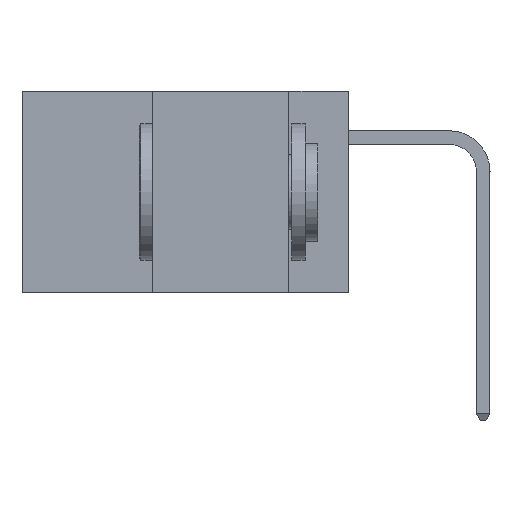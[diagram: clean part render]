
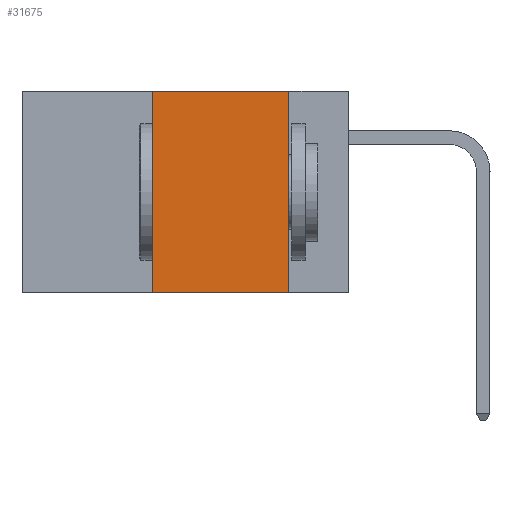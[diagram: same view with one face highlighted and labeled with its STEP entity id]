
A CAD part, left-side view. The second image highlights one B-rep face of the part: STEP entity #31675.
In plain terms, the highlighted planar face has unit normal (-1, 0, 0).
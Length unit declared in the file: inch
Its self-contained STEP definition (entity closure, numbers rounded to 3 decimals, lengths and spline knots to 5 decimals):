
#1002 = ORIENTED_EDGE ( 'NONE', *, *, #35847, .F. ) ;
#1972 = LINE ( 'NONE', #21958, #9373 ) ;
#2461 = LINE ( 'NONE', #11288, #18871 ) ;
#2498 = PLANE ( 'NONE',  #22065 ) ;
#6566 = CARTESIAN_POINT ( 'NONE',  ( 0., 0.36, -0.37 ) ) ;
#6732 = DIRECTION ( 'NONE',  ( 0., 0., -1. ) ) ;
#9373 = VECTOR ( 'NONE', #6732, 39.37008 ) ;
#9784 = VECTOR ( 'NONE', #36583, 39.37008 ) ;
#11142 = ORIENTED_EDGE ( 'NONE', *, *, #14828, .F. ) ;
#11288 = CARTESIAN_POINT ( 'NONE',  ( 0., 0.6, -0.37 ) ) ;
#11960 = DIRECTION ( 'NONE',  ( 0., 0., -1. ) ) ;
#13915 = CARTESIAN_POINT ( 'NONE',  ( 0., 0.36, 0. ) ) ;
#14675 = ORIENTED_EDGE ( 'NONE', *, *, #24342, .F. ) ;
#14828 = EDGE_CURVE ( 'NONE', #30409, #23588, #34005, .T. ) ;
#14893 = CARTESIAN_POINT ( 'NONE',  ( 0., 0.6, 0. ) ) ;
#16276 = DIRECTION ( 'NONE',  ( 0., 0., 1. ) ) ;
#17729 = VECTOR ( 'NONE', #16276, 39.37008 ) ;
#18871 = VECTOR ( 'NONE', #32500, 39.37008 ) ;
#19366 = CARTESIAN_POINT ( 'NONE',  ( 0., 0.11, -0.37 ) ) ;
#21958 = CARTESIAN_POINT ( 'NONE',  ( 0., 0.11, 0. ) ) ;
#22065 = AXIS2_PLACEMENT_3D ( 'NONE', #14893, #30103, #11960 ) ;
#23588 = VERTEX_POINT ( 'NONE', #36517 ) ;
#24342 = EDGE_CURVE ( 'NONE', #23588, #39618, #1972, .T. ) ;
#25503 = ORIENTED_EDGE ( 'NONE', *, *, #34550, .T. ) ;
#26681 = LINE ( 'NONE', #37509, #17729 ) ;
#27225 = EDGE_LOOP ( 'NONE', ( #14675, #11142, #1002, #25503 ) ) ;
#30103 = DIRECTION ( 'NONE',  ( 1., 0., 0. ) ) ;
#30409 = VERTEX_POINT ( 'NONE', #13915 ) ;
#31675 = ADVANCED_FACE ( 'NONE', ( #34331 ), #2498, .F. ) ;
#32500 = DIRECTION ( 'NONE',  ( 0., -1., 0. ) ) ;
#33507 = CARTESIAN_POINT ( 'NONE',  ( 0., 0.6, 0. ) ) ;
#33717 = VERTEX_POINT ( 'NONE', #6566 ) ;
#34005 = LINE ( 'NONE', #33507, #9784 ) ;
#34331 = FACE_OUTER_BOUND ( 'NONE', #27225, .T. ) ;
#34550 = EDGE_CURVE ( 'NONE', #33717, #39618, #2461, .T. ) ;
#35847 = EDGE_CURVE ( 'NONE', #33717, #30409, #26681, .T. ) ;
#36517 = CARTESIAN_POINT ( 'NONE',  ( 0., 0.11, 0. ) ) ;
#36583 = DIRECTION ( 'NONE',  ( 0., -1., 0. ) ) ;
#37509 = CARTESIAN_POINT ( 'NONE',  ( 0., 0.36, 0. ) ) ;
#39618 = VERTEX_POINT ( 'NONE', #19366 ) ;
